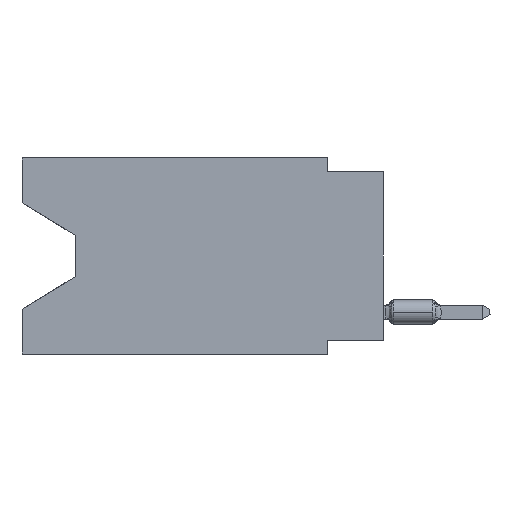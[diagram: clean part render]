
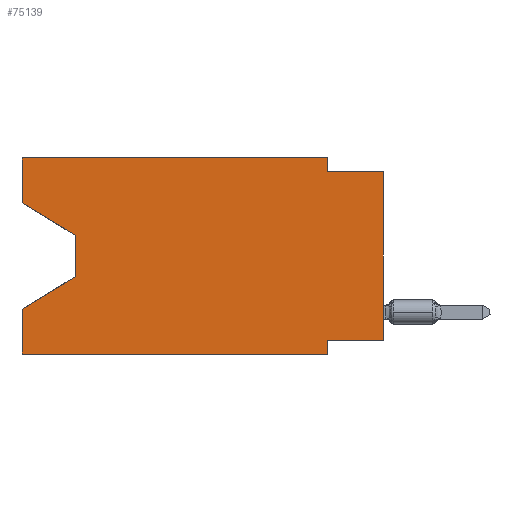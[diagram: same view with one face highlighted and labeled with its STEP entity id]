
A CAD part, left-side view. The second image highlights one B-rep face of the part: STEP entity #75139.
In plain terms, the highlighted planar face has unit normal (-1, 0, 0).
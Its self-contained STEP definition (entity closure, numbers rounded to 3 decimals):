
#110 = DIRECTION ( 'NONE',  ( 0., 0., 1. ) ) ;
#253 = ORIENTED_EDGE ( 'NONE', *, *, #23879, .F. ) ;
#636 = DIRECTION ( 'NONE',  ( 0., 0., -1. ) ) ;
#1154 = EDGE_CURVE ( 'NONE', #21396, #3267, #50803, .T. ) ;
#1448 = VERTEX_POINT ( 'NONE', #24821 ) ;
#1857 = EDGE_CURVE ( 'NONE', #65727, #4384, #4555, .T. ) ;
#2010 = EDGE_CURVE ( 'NONE', #4384, #8038, #20507, .T. ) ;
#2960 = CARTESIAN_POINT ( 'NONE',  ( 0., 2.54, 0. ) ) ;
#3267 = VERTEX_POINT ( 'NONE', #27354 ) ;
#3428 = CARTESIAN_POINT ( 'NONE',  ( 0., 2.54, -0.635 ) ) ;
#3723 = PLANE ( 'NONE',  #12469 ) ;
#4257 = DIRECTION ( 'NONE',  ( 0., 0., 1. ) ) ;
#4384 = VERTEX_POINT ( 'NONE', #59042 ) ;
#4555 = LINE ( 'NONE', #27817, #31688 ) ;
#4788 = EDGE_CURVE ( 'NONE', #21396, #66133, #24259, .T. ) ;
#5301 = VERTEX_POINT ( 'NONE', #65269 ) ;
#5648 = EDGE_CURVE ( 'NONE', #68194, #1448, #12532, .T. ) ;
#6351 = EDGE_CURVE ( 'NONE', #5301, #66133, #23437, .T. ) ;
#7033 = ORIENTED_EDGE ( 'NONE', *, *, #5648, .T. ) ;
#7217 = VECTOR ( 'NONE', #66284, 1000. ) ;
#7222 = ORIENTED_EDGE ( 'NONE', *, *, #6351, .F. ) ;
#7229 = VECTOR ( 'NONE', #4257, 1000. ) ;
#7549 = CARTESIAN_POINT ( 'NONE',  ( 0., 16.383, -2.038 ) ) ;
#8038 = VERTEX_POINT ( 'NONE', #3428 ) ;
#10034 = VECTOR ( 'NONE', #73640, 1000. ) ;
#11241 = CARTESIAN_POINT ( 'NONE',  ( 0., 2.54, -8.89 ) ) ;
#11327 = VECTOR ( 'NONE', #63767, 1000. ) ;
#11333 = CARTESIAN_POINT ( 'NONE',  ( 0., 16.383, 0. ) ) ;
#11625 = VECTOR ( 'NONE', #110, 1000. ) ;
#12469 = AXIS2_PLACEMENT_3D ( 'NONE', #11333, #17065, #636 ) ;
#12532 = LINE ( 'NONE', #59058, #59937 ) ;
#13604 = CARTESIAN_POINT ( 'NONE',  ( 0., 0., -8.255 ) ) ;
#14217 = CARTESIAN_POINT ( 'NONE',  ( 0., 16.383, 0. ) ) ;
#14965 = ORIENTED_EDGE ( 'NONE', *, *, #1857, .F. ) ;
#17065 = DIRECTION ( 'NONE',  ( 1., 0., 0. ) ) ;
#18260 = VERTEX_POINT ( 'NONE', #66666 ) ;
#20507 = LINE ( 'NONE', #2960, #48775 ) ;
#21396 = VERTEX_POINT ( 'NONE', #73652 ) ;
#23344 = LINE ( 'NONE', #33654, #11327 ) ;
#23374 = LINE ( 'NONE', #57701, #11625 ) ;
#23437 = LINE ( 'NONE', #11241, #63629 ) ;
#23879 = EDGE_CURVE ( 'NONE', #34828, #65727, #23374, .T. ) ;
#24259 = LINE ( 'NONE', #48285, #36732 ) ;
#24776 = ORIENTED_EDGE ( 'NONE', *, *, #28726, .T. ) ;
#24821 = CARTESIAN_POINT ( 'NONE',  ( 0., 0., -0.635 ) ) ;
#25631 = LINE ( 'NONE', #72532, #10034 ) ;
#26359 = CARTESIAN_POINT ( 'NONE',  ( 0., 0., -8.255 ) ) ;
#27354 = CARTESIAN_POINT ( 'NONE',  ( 0., 16.383, -6.852 ) ) ;
#27817 = CARTESIAN_POINT ( 'NONE',  ( 0., 16.383, 0. ) ) ;
#28726 = EDGE_CURVE ( 'NONE', #34828, #50614, #36520, .T. ) ;
#30220 = ORIENTED_EDGE ( 'NONE', *, *, #33039, .T. ) ;
#30984 = EDGE_CURVE ( 'NONE', #50614, #18260, #23344, .T. ) ;
#31688 = VECTOR ( 'NONE', #68654, 1000. ) ;
#31863 = ORIENTED_EDGE ( 'NONE', *, *, #1154, .F. ) ;
#33039 = EDGE_CURVE ( 'NONE', #18260, #3267, #25631, .T. ) ;
#33654 = CARTESIAN_POINT ( 'NONE',  ( 0., 13.97, -3.505 ) ) ;
#34497 = DIRECTION ( 'NONE',  ( 0., 0., -1. ) ) ;
#34828 = VERTEX_POINT ( 'NONE', #50677 ) ;
#34861 = EDGE_CURVE ( 'NONE', #8038, #1448, #70874, .T. ) ;
#34923 = CARTESIAN_POINT ( 'NONE',  ( 0., 13.97, -3.505 ) ) ;
#35315 = DIRECTION ( 'NONE',  ( 0., -1., 0. ) ) ;
#36520 = LINE ( 'NONE', #7549, #7217 ) ;
#36732 = VECTOR ( 'NONE', #35315, 1000. ) ;
#37809 = ORIENTED_EDGE ( 'NONE', *, *, #4788, .T. ) ;
#39204 = ORIENTED_EDGE ( 'NONE', *, *, #30984, .T. ) ;
#39773 = EDGE_CURVE ( 'NONE', #68194, #5301, #66238, .T. ) ;
#42634 = DIRECTION ( 'NONE',  ( 0., -1., 0. ) ) ;
#43302 = EDGE_LOOP ( 'NONE', ( #24776, #39204, #30220, #31863, #37809, #7222, #74401, #7033, #59694, #73820, #14965, #253 ) ) ;
#43770 = DIRECTION ( 'NONE',  ( 0., 0., -1. ) ) ;
#48285 = CARTESIAN_POINT ( 'NONE',  ( 0., 16.383, -8.89 ) ) ;
#48775 = VECTOR ( 'NONE', #43770, 1000. ) ;
#50614 = VERTEX_POINT ( 'NONE', #34923 ) ;
#50677 = CARTESIAN_POINT ( 'NONE',  ( 0., 16.383, -2.038 ) ) ;
#50803 = LINE ( 'NONE', #14217, #7229 ) ;
#52946 = CARTESIAN_POINT ( 'NONE',  ( 0., 0., -0.635 ) ) ;
#53649 = DIRECTION ( 'NONE',  ( 0., 1., 0. ) ) ;
#53722 = DIRECTION ( 'NONE',  ( 0., 0., 1. ) ) ;
#54579 = VECTOR ( 'NONE', #53649, 1000. ) ;
#55967 = FACE_OUTER_BOUND ( 'NONE', #43302, .T. ) ;
#57701 = CARTESIAN_POINT ( 'NONE',  ( 0., 16.383, 0. ) ) ;
#57787 = VECTOR ( 'NONE', #42634, 1000. ) ;
#59042 = CARTESIAN_POINT ( 'NONE',  ( 0., 2.54, 0. ) ) ;
#59058 = CARTESIAN_POINT ( 'NONE',  ( 0., 0., 0. ) ) ;
#59694 = ORIENTED_EDGE ( 'NONE', *, *, #34861, .F. ) ;
#59937 = VECTOR ( 'NONE', #53722, 1000. ) ;
#63629 = VECTOR ( 'NONE', #34497, 1000. ) ;
#63709 = CARTESIAN_POINT ( 'NONE',  ( 0., 16.383, 0. ) ) ;
#63767 = DIRECTION ( 'NONE',  ( 0., 0., -1. ) ) ;
#65269 = CARTESIAN_POINT ( 'NONE',  ( 0., 2.54, -8.255 ) ) ;
#65727 = VERTEX_POINT ( 'NONE', #63709 ) ;
#66133 = VERTEX_POINT ( 'NONE', #74689 ) ;
#66238 = LINE ( 'NONE', #13604, #54579 ) ;
#66284 = DIRECTION ( 'NONE',  ( 0., -0.855, -0.519 ) ) ;
#66666 = CARTESIAN_POINT ( 'NONE',  ( 0., 13.97, -5.385 ) ) ;
#68194 = VERTEX_POINT ( 'NONE', #26359 ) ;
#68654 = DIRECTION ( 'NONE',  ( 0., -1., 0. ) ) ;
#70874 = LINE ( 'NONE', #52946, #57787 ) ;
#72532 = CARTESIAN_POINT ( 'NONE',  ( 0., 13.97, -5.385 ) ) ;
#73640 = DIRECTION ( 'NONE',  ( 0., 0.855, -0.519 ) ) ;
#73652 = CARTESIAN_POINT ( 'NONE',  ( 0., 16.383, -8.89 ) ) ;
#73820 = ORIENTED_EDGE ( 'NONE', *, *, #2010, .F. ) ;
#74401 = ORIENTED_EDGE ( 'NONE', *, *, #39773, .F. ) ;
#74689 = CARTESIAN_POINT ( 'NONE',  ( 0., 2.54, -8.89 ) ) ;
#75139 = ADVANCED_FACE ( 'NONE', ( #55967 ), #3723, .F. ) ;
